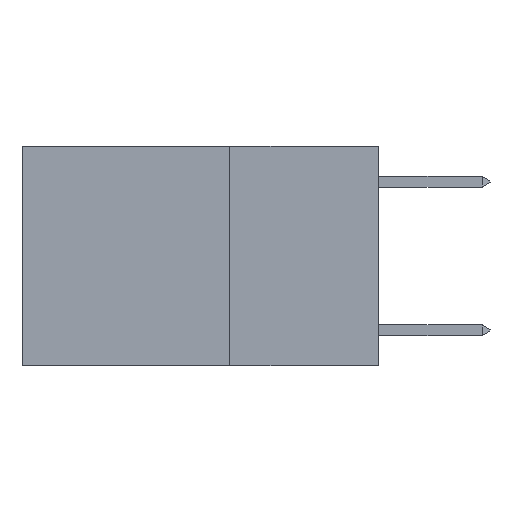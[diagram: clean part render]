
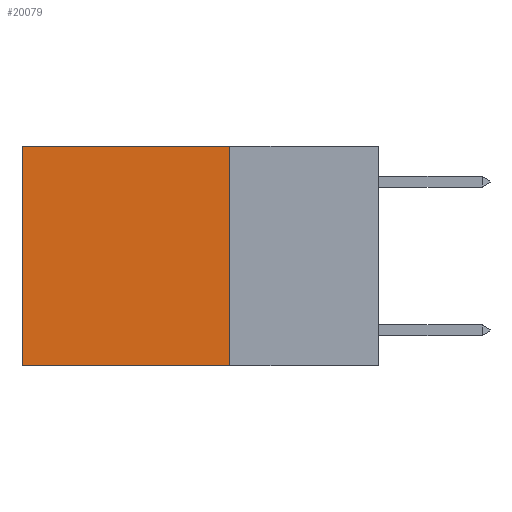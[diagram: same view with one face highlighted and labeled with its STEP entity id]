
A CAD part, left-side view. The second image highlights one B-rep face of the part: STEP entity #20079.
In plain terms, the highlighted planar face has unit normal (-1, 0, 0).
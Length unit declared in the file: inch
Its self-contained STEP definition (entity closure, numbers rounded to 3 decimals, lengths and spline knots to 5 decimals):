
#451 = LINE ( 'NONE', #6302, #14149 ) ;
#993 = PLANE ( 'NONE',  #10083 ) ;
#1114 = CARTESIAN_POINT ( 'NONE',  ( 0.2625, 0.25, 0. ) ) ;
#1118 = DIRECTION ( 'NONE',  ( 0., 1., 0. ) ) ;
#1765 = EDGE_LOOP ( 'NONE', ( #8659, #13116, #22010, #10993 ) ) ;
#2142 = VECTOR ( 'NONE', #2965, 39.37008 ) ;
#2159 = VERTEX_POINT ( 'NONE', #14116 ) ;
#2965 = DIRECTION ( 'NONE',  ( 0., 0., -1. ) ) ;
#3130 = FACE_OUTER_BOUND ( 'NONE', #1765, .T. ) ;
#4292 = VERTEX_POINT ( 'NONE', #22625 ) ;
#4444 = DIRECTION ( 'NONE',  ( 0., 0., -1. ) ) ;
#4567 = EDGE_CURVE ( 'NONE', #5939, #2159, #24032, .T. ) ;
#5712 = CARTESIAN_POINT ( 'NONE',  ( 0.2625, 0.25, 0. ) ) ;
#5939 = VERTEX_POINT ( 'NONE', #11116 ) ;
#6302 = CARTESIAN_POINT ( 'NONE',  ( 0.2625, 0.25, 0. ) ) ;
#6437 = EDGE_CURVE ( 'NONE', #4292, #21740, #17257, .T. ) ;
#7189 = DIRECTION ( 'NONE',  ( 1., 0., 0. ) ) ;
#8659 = ORIENTED_EDGE ( 'NONE', *, *, #4567, .T. ) ;
#10083 = AXIS2_PLACEMENT_3D ( 'NONE', #1114, #7189, #18247 ) ;
#10993 = ORIENTED_EDGE ( 'NONE', *, *, #20384, .T. ) ;
#11116 = CARTESIAN_POINT ( 'NONE',  ( 0.2625, 0.6, 0. ) ) ;
#12252 = DIRECTION ( 'NONE',  ( 0., 1., 0. ) ) ;
#12906 = CARTESIAN_POINT ( 'NONE',  ( 0.2625, 0.25, -0.37 ) ) ;
#13116 = ORIENTED_EDGE ( 'NONE', *, *, #16253, .F. ) ;
#13913 = VECTOR ( 'NONE', #4444, 39.37008 ) ;
#14116 = CARTESIAN_POINT ( 'NONE',  ( 0.2625, 0.6, -0.37 ) ) ;
#14149 = VECTOR ( 'NONE', #12252, 39.37008 ) ;
#16253 = EDGE_CURVE ( 'NONE', #21740, #2159, #18980, .T. ) ;
#17257 = LINE ( 'NONE', #5712, #2142 ) ;
#17656 = VECTOR ( 'NONE', #1118, 39.37008 ) ;
#17710 = CARTESIAN_POINT ( 'NONE',  ( 0.2625, 0.25, -0.37 ) ) ;
#18247 = DIRECTION ( 'NONE',  ( 0., 0., -1. ) ) ;
#18980 = LINE ( 'NONE', #12906, #17656 ) ;
#20079 = ADVANCED_FACE ( 'NONE', ( #3130 ), #993, .F. ) ;
#20384 = EDGE_CURVE ( 'NONE', #4292, #5939, #451, .T. ) ;
#21740 = VERTEX_POINT ( 'NONE', #17710 ) ;
#22010 = ORIENTED_EDGE ( 'NONE', *, *, #6437, .F. ) ;
#22625 = CARTESIAN_POINT ( 'NONE',  ( 0.2625, 0.25, 0. ) ) ;
#23655 = CARTESIAN_POINT ( 'NONE',  ( 0.2625, 0.6, 0. ) ) ;
#24032 = LINE ( 'NONE', #23655, #13913 ) ;
